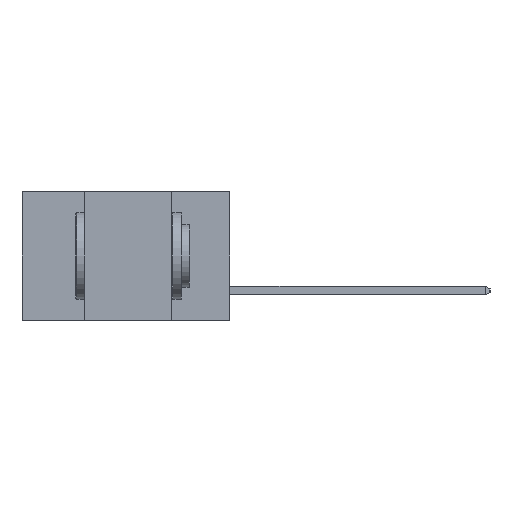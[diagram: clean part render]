
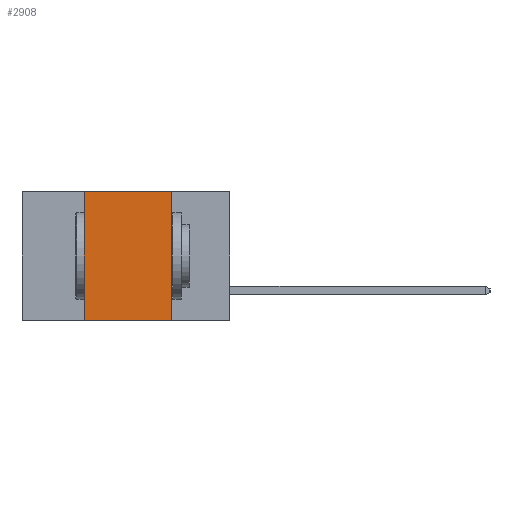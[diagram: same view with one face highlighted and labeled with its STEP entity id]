
A CAD part, left-side view. The second image highlights one B-rep face of the part: STEP entity #2908.
In plain terms, the highlighted planar face has unit normal (-1, 0, 0).
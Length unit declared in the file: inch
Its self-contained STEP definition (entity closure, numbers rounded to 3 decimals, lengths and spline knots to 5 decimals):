
#66 = CARTESIAN_POINT ( 'NONE',  ( 0., 0.42, 0. ) ) ;
#523 = AXIS2_PLACEMENT_3D ( 'NONE', #756, #4821, #15351 ) ;
#756 = CARTESIAN_POINT ( 'NONE',  ( 0., 0.6, 0. ) ) ;
#1858 = VERTEX_POINT ( 'NONE', #66 ) ;
#1958 = CARTESIAN_POINT ( 'NONE',  ( 0., 0.42, -0.37 ) ) ;
#2159 = CARTESIAN_POINT ( 'NONE',  ( 0., 0.17, -0.37 ) ) ;
#2908 = ADVANCED_FACE ( 'NONE', ( #9551 ), #14170, .F. ) ;
#2919 = CARTESIAN_POINT ( 'NONE',  ( 0., 0.42, -0.37 ) ) ;
#3946 = EDGE_CURVE ( 'NONE', #1858, #12464, #18196, .T. ) ;
#4582 = VECTOR ( 'NONE', #15923, 39.37008 ) ;
#4821 = DIRECTION ( 'NONE',  ( 1., 0., 0. ) ) ;
#5469 = VECTOR ( 'NONE', #16779, 39.37008 ) ;
#6802 = VECTOR ( 'NONE', #14868, 39.37008 ) ;
#7599 = VERTEX_POINT ( 'NONE', #2159 ) ;
#7606 = ORIENTED_EDGE ( 'NONE', *, *, #15231, .F. ) ;
#7620 = ORIENTED_EDGE ( 'NONE', *, *, #3946, .F. ) ;
#7628 = VERTEX_POINT ( 'NONE', #1958 ) ;
#8106 = ORIENTED_EDGE ( 'NONE', *, *, #14862, .F. ) ;
#8165 = EDGE_LOOP ( 'NONE', ( #7606, #7620, #8106, #8468 ) ) ;
#8445 = LINE ( 'NONE', #2919, #4582 ) ;
#8468 = ORIENTED_EDGE ( 'NONE', *, *, #13389, .T. ) ;
#9551 = FACE_OUTER_BOUND ( 'NONE', #8165, .T. ) ;
#10494 = LINE ( 'NONE', #13614, #17638 ) ;
#12464 = VERTEX_POINT ( 'NONE', #13834 ) ;
#13389 = EDGE_CURVE ( 'NONE', #7628, #7599, #10494, .T. ) ;
#13614 = CARTESIAN_POINT ( 'NONE',  ( 0., 0.6, -0.37 ) ) ;
#13706 = DIRECTION ( 'NONE',  ( 0., -1., 0. ) ) ;
#13834 = CARTESIAN_POINT ( 'NONE',  ( 0., 0.17, 0. ) ) ;
#14170 = PLANE ( 'NONE',  #523 ) ;
#14554 = LINE ( 'NONE', #18141, #5469 ) ;
#14835 = CARTESIAN_POINT ( 'NONE',  ( 0., 0.6, 0. ) ) ;
#14862 = EDGE_CURVE ( 'NONE', #7628, #1858, #8445, .T. ) ;
#14868 = DIRECTION ( 'NONE',  ( 0., -1., 0. ) ) ;
#15231 = EDGE_CURVE ( 'NONE', #12464, #7599, #14554, .T. ) ;
#15351 = DIRECTION ( 'NONE',  ( 0., 0., -1. ) ) ;
#15923 = DIRECTION ( 'NONE',  ( 0., 0., 1. ) ) ;
#16779 = DIRECTION ( 'NONE',  ( 0., 0., -1. ) ) ;
#17638 = VECTOR ( 'NONE', #13706, 39.37008 ) ;
#18141 = CARTESIAN_POINT ( 'NONE',  ( 0., 0.17, -0.37 ) ) ;
#18196 = LINE ( 'NONE', #14835, #6802 ) ;
